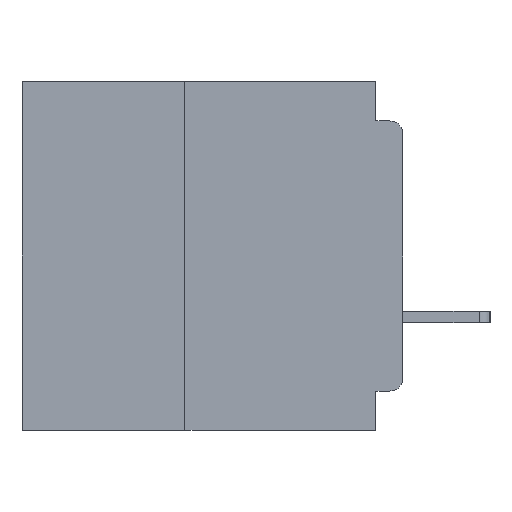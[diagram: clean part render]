
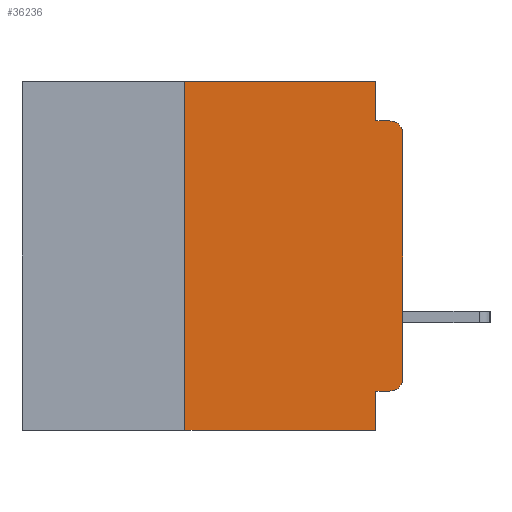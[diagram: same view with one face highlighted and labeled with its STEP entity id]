
A CAD part, left-side view. The second image highlights one B-rep face of the part: STEP entity #36236.
In plain terms, the highlighted planar face has unit normal (-1, 0, 0).
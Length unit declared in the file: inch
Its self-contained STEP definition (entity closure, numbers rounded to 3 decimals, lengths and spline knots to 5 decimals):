
#29 = CARTESIAN_POINT ( 'NONE',  ( 0., 0., -0.06 ) ) ;
#181 = ORIENTED_EDGE ( 'NONE', *, *, #21632, .T. ) ;
#357 = VECTOR ( 'NONE', #18906, 39.37008 ) ;
#422 = VECTOR ( 'NONE', #35628, 39.37008 ) ;
#2851 = VECTOR ( 'NONE', #8691, 39.37008 ) ;
#3150 = DIRECTION ( 'NONE',  ( 0., -1., 0. ) ) ;
#3508 = CARTESIAN_POINT ( 'NONE',  ( 0., 0.437, 0. ) ) ;
#4566 = CARTESIAN_POINT ( 'NONE',  ( 0., 0.25, 0. ) ) ;
#5379 = CARTESIAN_POINT ( 'NONE',  ( 0., 0.031, 0. ) ) ;
#6610 = FACE_OUTER_BOUND ( 'NONE', #30218, .T. ) ;
#7115 = ORIENTED_EDGE ( 'NONE', *, *, #36031, .F. ) ;
#7218 = CARTESIAN_POINT ( 'NONE',  ( 0., 0., -0.355 ) ) ;
#8026 = DIRECTION ( 'NONE',  ( 0., 0., -1. ) ) ;
#8466 = ORIENTED_EDGE ( 'NONE', *, *, #38169, .T. ) ;
#8691 = DIRECTION ( 'NONE',  ( 0., -1., 0. ) ) ;
#9613 = ORIENTED_EDGE ( 'NONE', *, *, #11392, .F. ) ;
#9734 = EDGE_CURVE ( 'NONE', #12111, #15796, #50099, .T. ) ;
#10797 = EDGE_CURVE ( 'NONE', #23958, #43975, #20990, .T. ) ;
#11113 = DIRECTION ( 'NONE',  ( -1., 0., 0. ) ) ;
#11392 = EDGE_CURVE ( 'NONE', #43975, #44943, #20297, .T. ) ;
#12111 = VERTEX_POINT ( 'NONE', #17348 ) ;
#13778 = CARTESIAN_POINT ( 'NONE',  ( 0., 0.015, -0.355 ) ) ;
#15228 = CARTESIAN_POINT ( 'NONE',  ( 0., 0.25, -0.4 ) ) ;
#15796 = VERTEX_POINT ( 'NONE', #29 ) ;
#16503 = VERTEX_POINT ( 'NONE', #49565 ) ;
#17348 = CARTESIAN_POINT ( 'NONE',  ( 0., 0., -0.34 ) ) ;
#18039 = DIRECTION ( 'NONE',  ( -1., 0., 0. ) ) ;
#18503 = CARTESIAN_POINT ( 'NONE',  ( 0., 0.25, -0.4 ) ) ;
#18906 = DIRECTION ( 'NONE',  ( 0., 0., -1. ) ) ;
#19916 = VERTEX_POINT ( 'NONE', #45377 ) ;
#20098 = DIRECTION ( 'NONE',  ( 0., 0., -1. ) ) ;
#20297 = LINE ( 'NONE', #31738, #41659 ) ;
#20874 = ORIENTED_EDGE ( 'NONE', *, *, #9734, .T. ) ;
#20990 = LINE ( 'NONE', #27005, #357 ) ;
#21632 = EDGE_CURVE ( 'NONE', #15796, #44943, #43312, .T. ) ;
#22127 = ORIENTED_EDGE ( 'NONE', *, *, #51436, .F. ) ;
#22665 = VECTOR ( 'NONE', #8026, 39.37008 ) ;
#23729 = ORIENTED_EDGE ( 'NONE', *, *, #39344, .F. ) ;
#23958 = VERTEX_POINT ( 'NONE', #5379 ) ;
#24559 = ORIENTED_EDGE ( 'NONE', *, *, #37025, .F. ) ;
#26657 = ORIENTED_EDGE ( 'NONE', *, *, #33652, .T. ) ;
#27005 = CARTESIAN_POINT ( 'NONE',  ( 0., 0.031, 0. ) ) ;
#27375 = CIRCLE ( 'NONE', #39969, 0.015 ) ;
#28688 = VECTOR ( 'NONE', #52703, 39.37008 ) ;
#28800 = VERTEX_POINT ( 'NONE', #15228 ) ;
#29012 = CARTESIAN_POINT ( 'NONE',  ( 0., 0.437, -0.4 ) ) ;
#29524 = LINE ( 'NONE', #33680, #37643 ) ;
#30218 = EDGE_LOOP ( 'NONE', ( #20874, #181, #9613, #44842, #24559, #7115, #8466, #23729, #22127, #26657 ) ) ;
#31738 = CARTESIAN_POINT ( 'NONE',  ( 0., 0., -0.045 ) ) ;
#31784 = LINE ( 'NONE', #7218, #422 ) ;
#32142 = LINE ( 'NONE', #32415, #22665 ) ;
#32415 = CARTESIAN_POINT ( 'NONE',  ( 0., 0.031, -0.4 ) ) ;
#32588 = CARTESIAN_POINT ( 'NONE',  ( 0., 0., 0. ) ) ;
#33652 = EDGE_CURVE ( 'NONE', #43677, #12111, #27375, .T. ) ;
#33680 = CARTESIAN_POINT ( 'NONE',  ( 0., 0.437, 0. ) ) ;
#34893 = CARTESIAN_POINT ( 'NONE',  ( 0., 0.015, -0.045 ) ) ;
#35377 = CARTESIAN_POINT ( 'NONE',  ( 0., 0.015, -0.06 ) ) ;
#35628 = DIRECTION ( 'NONE',  ( 0., 1., 0. ) ) ;
#36031 = EDGE_CURVE ( 'NONE', #28800, #36395, #40928, .T. ) ;
#36236 = ADVANCED_FACE ( 'NONE', ( #6610 ), #40118, .F. ) ;
#36395 = VERTEX_POINT ( 'NONE', #4566 ) ;
#36615 = LINE ( 'NONE', #29012, #2851 ) ;
#37025 = EDGE_CURVE ( 'NONE', #36395, #23958, #29524, .T. ) ;
#37643 = VECTOR ( 'NONE', #37689, 39.37008 ) ;
#37689 = DIRECTION ( 'NONE',  ( 0., -1., 0. ) ) ;
#38169 = EDGE_CURVE ( 'NONE', #28800, #19916, #36615, .T. ) ;
#38391 = VECTOR ( 'NONE', #46675, 39.37008 ) ;
#39182 = AXIS2_PLACEMENT_3D ( 'NONE', #35377, #11113, #39415 ) ;
#39344 = EDGE_CURVE ( 'NONE', #16503, #19916, #32142, .T. ) ;
#39415 = DIRECTION ( 'NONE',  ( 0., 0., -1. ) ) ;
#39884 = CARTESIAN_POINT ( 'NONE',  ( 0., 0.031, -0.045 ) ) ;
#39969 = AXIS2_PLACEMENT_3D ( 'NONE', #42140, #18039, #46199 ) ;
#40118 = PLANE ( 'NONE',  #51850 ) ;
#40928 = LINE ( 'NONE', #18503, #38391 ) ;
#41659 = VECTOR ( 'NONE', #3150, 39.37008 ) ;
#42140 = CARTESIAN_POINT ( 'NONE',  ( 0., 0.015, -0.34 ) ) ;
#43312 = CIRCLE ( 'NONE', #39182, 0.015 ) ;
#43677 = VERTEX_POINT ( 'NONE', #13778 ) ;
#43975 = VERTEX_POINT ( 'NONE', #39884 ) ;
#44182 = DIRECTION ( 'NONE',  ( 1., 0., 0. ) ) ;
#44842 = ORIENTED_EDGE ( 'NONE', *, *, #10797, .F. ) ;
#44943 = VERTEX_POINT ( 'NONE', #34893 ) ;
#45377 = CARTESIAN_POINT ( 'NONE',  ( 0., 0.031, -0.4 ) ) ;
#46199 = DIRECTION ( 'NONE',  ( 0., 0., -1. ) ) ;
#46675 = DIRECTION ( 'NONE',  ( 0., 0., 1. ) ) ;
#49565 = CARTESIAN_POINT ( 'NONE',  ( 0., 0.031, -0.355 ) ) ;
#50099 = LINE ( 'NONE', #32588, #28688 ) ;
#51436 = EDGE_CURVE ( 'NONE', #43677, #16503, #31784, .T. ) ;
#51850 = AXIS2_PLACEMENT_3D ( 'NONE', #3508, #44182, #20098 ) ;
#52703 = DIRECTION ( 'NONE',  ( 0., 0., 1. ) ) ;
